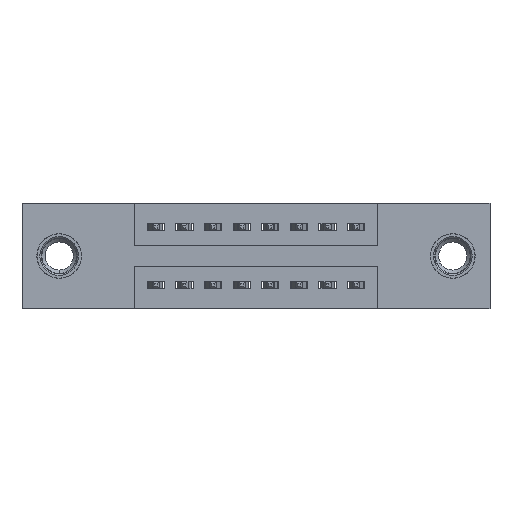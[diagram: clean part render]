
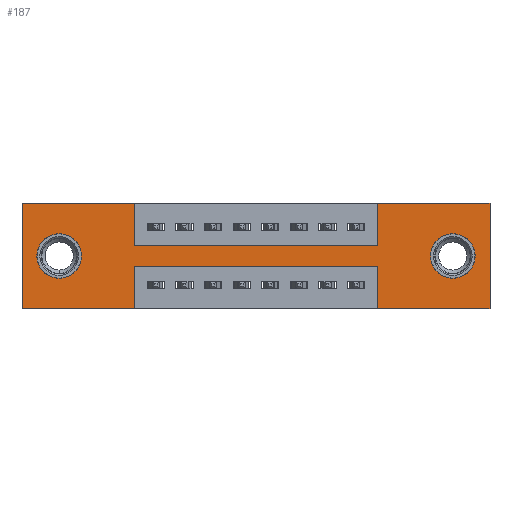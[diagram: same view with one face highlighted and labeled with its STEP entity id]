
A CAD part, front view. The second image highlights one B-rep face of the part: STEP entity #187.
In plain terms, the highlighted planar face has unit normal (0, -1, 0).
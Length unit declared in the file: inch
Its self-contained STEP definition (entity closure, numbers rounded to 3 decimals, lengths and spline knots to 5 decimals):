
#4 = VECTOR ( 'NONE', #316, 39.37008 ) ;
#62 = ORIENTED_EDGE ( 'NONE', *, *, #1828, .F. ) ;
#122 = FACE_OUTER_BOUND ( 'NONE', #11455, .T. ) ;
#187 = ADVANCED_FACE ( 'NONE', ( #426, #9907, #122 ), #1323, .T. ) ;
#283 = VECTOR ( 'NONE', #535, 39.37008 ) ;
#302 = EDGE_CURVE ( 'NONE', #440, #1097, #1463, .T. ) ;
#316 = DIRECTION ( 'NONE',  ( 0., 0., 1. ) ) ;
#367 = EDGE_CURVE ( 'NONE', #4734, #6265, #3096, .T. ) ;
#402 = CARTESIAN_POINT ( 'NONE',  ( 0., 0., -0.37 ) ) ;
#426 = FACE_BOUND ( 'NONE', #4008, .T. ) ;
#440 = VERTEX_POINT ( 'NONE', #8362 ) ;
#495 = CARTESIAN_POINT ( 'NONE',  ( 0.13, 0., -0.107 ) ) ;
#507 = ORIENTED_EDGE ( 'NONE', *, *, #3165, .F. ) ;
#535 = DIRECTION ( 'NONE',  ( 1., 0., 0. ) ) ;
#565 = VECTOR ( 'NONE', #9361, 39.37008 ) ;
#576 = DIRECTION ( 'NONE',  ( 0., 0., 1. ) ) ;
#712 = EDGE_CURVE ( 'NONE', #8742, #11922, #4830, .T. ) ;
#774 = CARTESIAN_POINT ( 'NONE',  ( 1.635, 0., -0.37 ) ) ;
#988 = EDGE_CURVE ( 'NONE', #3489, #9712, #6579, .T. ) ;
#1048 = CARTESIAN_POINT ( 'NONE',  ( 0.3925, 0., 0. ) ) ;
#1097 = VERTEX_POINT ( 'NONE', #9515 ) ;
#1175 = DIRECTION ( 'NONE',  ( 0., 0., -1. ) ) ;
#1249 = VERTEX_POINT ( 'NONE', #10148 ) ;
#1254 = DIRECTION ( 'NONE',  ( 0., 1., 0. ) ) ;
#1293 = EDGE_CURVE ( 'NONE', #6265, #5350, #5824, .T. ) ;
#1323 = PLANE ( 'NONE',  #7260 ) ;
#1358 = LINE ( 'NONE', #8000, #11030 ) ;
#1463 = LINE ( 'NONE', #8385, #6147 ) ;
#1491 = CARTESIAN_POINT ( 'NONE',  ( 0., 0., 0. ) ) ;
#1572 = EDGE_CURVE ( 'NONE', #8320, #6790, #10153, .T. ) ;
#1583 = CARTESIAN_POINT ( 'NONE',  ( 0., 0., -0.37 ) ) ;
#1639 = CARTESIAN_POINT ( 'NONE',  ( 0., 0., 0. ) ) ;
#1792 = VERTEX_POINT ( 'NONE', #9459 ) ;
#1828 = EDGE_CURVE ( 'NONE', #11922, #3078, #10288, .T. ) ;
#1851 = VERTEX_POINT ( 'NONE', #7908 ) ;
#1997 = ORIENTED_EDGE ( 'NONE', *, *, #5590, .F. ) ;
#2050 = AXIS2_PLACEMENT_3D ( 'NONE', #6877, #1254, #7842 ) ;
#2590 = ORIENTED_EDGE ( 'NONE', *, *, #712, .F. ) ;
#2722 = VECTOR ( 'NONE', #2975, 39.37008 ) ;
#2793 = DIRECTION ( 'NONE',  ( 0., 0., 1. ) ) ;
#2835 = LINE ( 'NONE', #5939, #4 ) ;
#2975 = DIRECTION ( 'NONE',  ( 0., 0., -1. ) ) ;
#3078 = VERTEX_POINT ( 'NONE', #3737 ) ;
#3096 = LINE ( 'NONE', #402, #565 ) ;
#3128 = CARTESIAN_POINT ( 'NONE',  ( 0.3925, 0., -0.37 ) ) ;
#3165 = EDGE_CURVE ( 'NONE', #1097, #4734, #10524, .T. ) ;
#3326 = ORIENTED_EDGE ( 'NONE', *, *, #5503, .F. ) ;
#3353 = VECTOR ( 'NONE', #2793, 39.37008 ) ;
#3489 = VERTEX_POINT ( 'NONE', #774 ) ;
#3737 = CARTESIAN_POINT ( 'NONE',  ( 1.2425, 0., -0.15 ) ) ;
#3754 = DIRECTION ( 'NONE',  ( 0., 0., 1. ) ) ;
#3842 = EDGE_CURVE ( 'NONE', #1792, #1249, #4028, .T. ) ;
#4008 = EDGE_LOOP ( 'NONE', ( #7119, #9706 ) ) ;
#4028 = CIRCLE ( 'NONE', #9973, 0.078 ) ;
#4094 = VECTOR ( 'NONE', #11985, 39.37008 ) ;
#4496 = ORIENTED_EDGE ( 'NONE', *, *, #6829, .F. ) ;
#4734 = VERTEX_POINT ( 'NONE', #4861 ) ;
#4779 = DIRECTION ( 'NONE',  ( 0., 1., 0. ) ) ;
#4810 = EDGE_CURVE ( 'NONE', #1249, #1792, #8024, .T. ) ;
#4830 = LINE ( 'NONE', #1048, #11667 ) ;
#4861 = CARTESIAN_POINT ( 'NONE',  ( 0.3925, 0., -0.37 ) ) ;
#5350 = VERTEX_POINT ( 'NONE', #6692 ) ;
#5368 = ORIENTED_EDGE ( 'NONE', *, *, #367, .F. ) ;
#5503 = EDGE_CURVE ( 'NONE', #9712, #440, #2835, .T. ) ;
#5528 = VECTOR ( 'NONE', #8325, 39.37008 ) ;
#5590 = EDGE_CURVE ( 'NONE', #1851, #3489, #1358, .T. ) ;
#5606 = EDGE_LOOP ( 'NONE', ( #7416, #10263 ) ) ;
#5746 = CARTESIAN_POINT ( 'NONE',  ( 0.13, 0., -0.185 ) ) ;
#5824 = LINE ( 'NONE', #1639, #3353 ) ;
#5939 = CARTESIAN_POINT ( 'NONE',  ( 1.2425, 0., -0.37 ) ) ;
#6011 = VECTOR ( 'NONE', #6554, 39.37008 ) ;
#6033 = VECTOR ( 'NONE', #10278, 39.37008 ) ;
#6091 = ORIENTED_EDGE ( 'NONE', *, *, #988, .F. ) ;
#6147 = VECTOR ( 'NONE', #8538, 39.37008 ) ;
#6199 = DIRECTION ( 'NONE',  ( 0., 1., 0. ) ) ;
#6265 = VERTEX_POINT ( 'NONE', #1583 ) ;
#6554 = DIRECTION ( 'NONE',  ( 0., 0., 1. ) ) ;
#6579 = LINE ( 'NONE', #12002, #4094 ) ;
#6611 = LINE ( 'NONE', #9414, #6011 ) ;
#6692 = CARTESIAN_POINT ( 'NONE',  ( 0., 0., 0. ) ) ;
#6790 = VERTEX_POINT ( 'NONE', #495 ) ;
#6829 = EDGE_CURVE ( 'NONE', #9921, #1851, #7491, .T. ) ;
#6837 = EDGE_CURVE ( 'NONE', #6790, #8320, #9772, .T. ) ;
#6877 = CARTESIAN_POINT ( 'NONE',  ( 1.505, 0., -0.185 ) ) ;
#6941 = AXIS2_PLACEMENT_3D ( 'NONE', #11760, #6199, #576 ) ;
#7119 = ORIENTED_EDGE ( 'NONE', *, *, #3842, .T. ) ;
#7260 = AXIS2_PLACEMENT_3D ( 'NONE', #10896, #9265, #8604 ) ;
#7416 = ORIENTED_EDGE ( 'NONE', *, *, #6837, .T. ) ;
#7491 = LINE ( 'NONE', #1491, #283 ) ;
#7586 = ORIENTED_EDGE ( 'NONE', *, *, #10053, .F. ) ;
#7682 = LINE ( 'NONE', #11150, #6033 ) ;
#7842 = DIRECTION ( 'NONE',  ( 0., 0., -1. ) ) ;
#7908 = CARTESIAN_POINT ( 'NONE',  ( 1.635, 0., 0. ) ) ;
#8000 = CARTESIAN_POINT ( 'NONE',  ( 1.635, 0., 0. ) ) ;
#8024 = CIRCLE ( 'NONE', #2050, 0.078 ) ;
#8228 = DIRECTION ( 'NONE',  ( 0., 0., -1. ) ) ;
#8269 = DIRECTION ( 'NONE',  ( 0., 1., 0. ) ) ;
#8285 = CARTESIAN_POINT ( 'NONE',  ( 1.505, 0., -0.185 ) ) ;
#8288 = CARTESIAN_POINT ( 'NONE',  ( 0.3925, 0., -0.15 ) ) ;
#8320 = VERTEX_POINT ( 'NONE', #11884 ) ;
#8325 = DIRECTION ( 'NONE',  ( 1., 0., 0. ) ) ;
#8362 = CARTESIAN_POINT ( 'NONE',  ( 1.2425, 0., -0.22 ) ) ;
#8385 = CARTESIAN_POINT ( 'NONE',  ( 0.3925, 0., -0.22 ) ) ;
#8538 = DIRECTION ( 'NONE',  ( -1., 0., 0. ) ) ;
#8604 = DIRECTION ( 'NONE',  ( 0., 0., -1. ) ) ;
#8742 = VERTEX_POINT ( 'NONE', #8912 ) ;
#8884 = CARTESIAN_POINT ( 'NONE',  ( 1.2425, 0., 0. ) ) ;
#8912 = CARTESIAN_POINT ( 'NONE',  ( 0.3925, 0., 0. ) ) ;
#8936 = DIRECTION ( 'NONE',  ( 0., 0., -1. ) ) ;
#9265 = DIRECTION ( 'NONE',  ( 0., -1., 0. ) ) ;
#9361 = DIRECTION ( 'NONE',  ( -1., 0., 0. ) ) ;
#9387 = CARTESIAN_POINT ( 'NONE',  ( 0.3925, 0., -0.15 ) ) ;
#9414 = CARTESIAN_POINT ( 'NONE',  ( 1.2425, 0., 0. ) ) ;
#9459 = CARTESIAN_POINT ( 'NONE',  ( 1.505, 0., -0.107 ) ) ;
#9515 = CARTESIAN_POINT ( 'NONE',  ( 0.3925, 0., -0.22 ) ) ;
#9706 = ORIENTED_EDGE ( 'NONE', *, *, #4810, .T. ) ;
#9712 = VERTEX_POINT ( 'NONE', #11294 ) ;
#9772 = CIRCLE ( 'NONE', #6941, 0.078 ) ;
#9856 = ORIENTED_EDGE ( 'NONE', *, *, #10720, .F. ) ;
#9907 = FACE_BOUND ( 'NONE', #5606, .T. ) ;
#9921 = VERTEX_POINT ( 'NONE', #8884 ) ;
#9973 = AXIS2_PLACEMENT_3D ( 'NONE', #8285, #8269, #8228 ) ;
#10053 = EDGE_CURVE ( 'NONE', #5350, #8742, #7682, .T. ) ;
#10130 = ORIENTED_EDGE ( 'NONE', *, *, #1293, .F. ) ;
#10148 = CARTESIAN_POINT ( 'NONE',  ( 1.505, 0., -0.263 ) ) ;
#10153 = CIRCLE ( 'NONE', #10164, 0.078 ) ;
#10164 = AXIS2_PLACEMENT_3D ( 'NONE', #5746, #4779, #3754 ) ;
#10263 = ORIENTED_EDGE ( 'NONE', *, *, #1572, .T. ) ;
#10278 = DIRECTION ( 'NONE',  ( 1., 0., 0. ) ) ;
#10288 = LINE ( 'NONE', #8288, #5528 ) ;
#10524 = LINE ( 'NONE', #3128, #2722 ) ;
#10534 = ORIENTED_EDGE ( 'NONE', *, *, #302, .F. ) ;
#10720 = EDGE_CURVE ( 'NONE', #3078, #9921, #6611, .T. ) ;
#10896 = CARTESIAN_POINT ( 'NONE',  ( 0., 0., -0.37 ) ) ;
#11030 = VECTOR ( 'NONE', #8936, 39.37008 ) ;
#11150 = CARTESIAN_POINT ( 'NONE',  ( 0., 0., 0. ) ) ;
#11294 = CARTESIAN_POINT ( 'NONE',  ( 1.2425, 0., -0.37 ) ) ;
#11455 = EDGE_LOOP ( 'NONE', ( #507, #10534, #3326, #6091, #1997, #4496, #9856, #62, #2590, #7586, #10130, #5368 ) ) ;
#11667 = VECTOR ( 'NONE', #1175, 39.37008 ) ;
#11760 = CARTESIAN_POINT ( 'NONE',  ( 0.13, 0., -0.185 ) ) ;
#11884 = CARTESIAN_POINT ( 'NONE',  ( 0.13, 0., -0.263 ) ) ;
#11922 = VERTEX_POINT ( 'NONE', #9387 ) ;
#11985 = DIRECTION ( 'NONE',  ( -1., 0., 0. ) ) ;
#12002 = CARTESIAN_POINT ( 'NONE',  ( 0., 0., -0.37 ) ) ;
